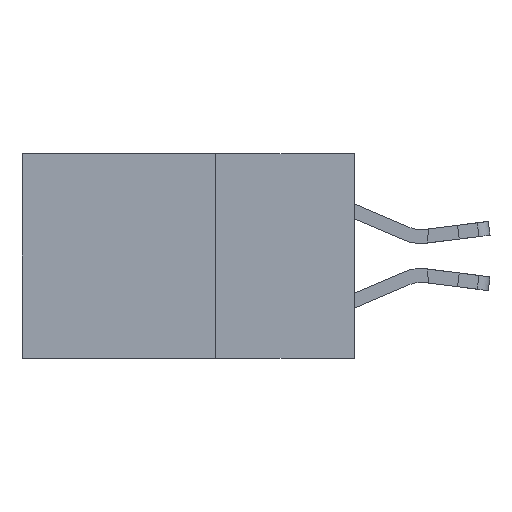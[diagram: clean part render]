
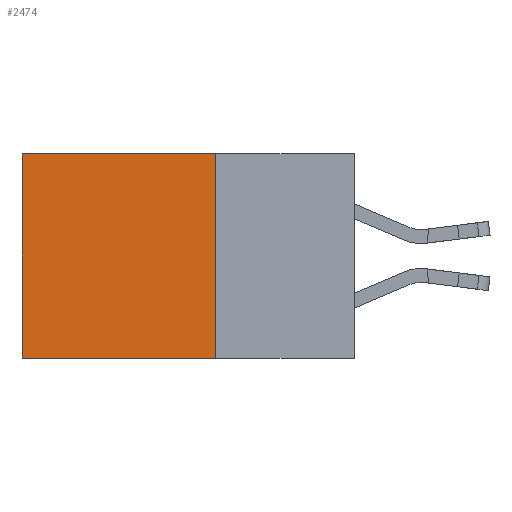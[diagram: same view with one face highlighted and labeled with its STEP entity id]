
A CAD part, left-side view. The second image highlights one B-rep face of the part: STEP entity #2474.
In plain terms, the highlighted planar face has unit normal (-1, 0, 0).
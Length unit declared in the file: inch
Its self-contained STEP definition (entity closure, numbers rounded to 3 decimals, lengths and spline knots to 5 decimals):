
#493 = CARTESIAN_POINT ( 'NONE',  ( 0.298, 0.25, 0. ) ) ;
#2474 = ADVANCED_FACE ( 'NONE', ( #22969 ), #17790, .F. ) ;
#2578 = VERTEX_POINT ( 'NONE', #23545 ) ;
#2821 = VERTEX_POINT ( 'NONE', #23646 ) ;
#2995 = DIRECTION ( 'NONE',  ( 0., 1., 0. ) ) ;
#3451 = AXIS2_PLACEMENT_3D ( 'NONE', #17655, #21585, #21608 ) ;
#4614 = ORIENTED_EDGE ( 'NONE', *, *, #14174, .F. ) ;
#4644 = DIRECTION ( 'NONE',  ( 0., 0., -1. ) ) ;
#5321 = CARTESIAN_POINT ( 'NONE',  ( 0.298, 0.25, 0. ) ) ;
#5442 = LINE ( 'NONE', #5321, #15656 ) ;
#6389 = VECTOR ( 'NONE', #17091, 39.37008 ) ;
#7253 = EDGE_CURVE ( 'NONE', #2821, #21787, #18313, .T. ) ;
#8786 = VECTOR ( 'NONE', #4644, 39.37008 ) ;
#9282 = EDGE_CURVE ( 'NONE', #15193, #2821, #17267, .T. ) ;
#11605 = EDGE_LOOP ( 'NONE', ( #11889, #17019, #4614, #24381 ) ) ;
#11856 = VECTOR ( 'NONE', #2995, 39.37008 ) ;
#11889 = ORIENTED_EDGE ( 'NONE', *, *, #7253, .T. ) ;
#12897 = CARTESIAN_POINT ( 'NONE',  ( 0.298, 0.25, 0. ) ) ;
#14174 = EDGE_CURVE ( 'NONE', #15193, #2578, #5442, .T. ) ;
#15193 = VERTEX_POINT ( 'NONE', #493 ) ;
#15656 = VECTOR ( 'NONE', #23726, 39.37008 ) ;
#16890 = CARTESIAN_POINT ( 'NONE',  ( 0.298, 0.6, 0. ) ) ;
#17019 = ORIENTED_EDGE ( 'NONE', *, *, #21479, .F. ) ;
#17091 = DIRECTION ( 'NONE',  ( 0., 1., 0. ) ) ;
#17267 = LINE ( 'NONE', #12897, #6389 ) ;
#17308 = LINE ( 'NONE', #25360, #11856 ) ;
#17655 = CARTESIAN_POINT ( 'NONE',  ( 0.298, 0.25, 0. ) ) ;
#17790 = PLANE ( 'NONE',  #3451 ) ;
#18162 = CARTESIAN_POINT ( 'NONE',  ( 0.298, 0.6, -0.37 ) ) ;
#18313 = LINE ( 'NONE', #16890, #8786 ) ;
#21479 = EDGE_CURVE ( 'NONE', #2578, #21787, #17308, .T. ) ;
#21585 = DIRECTION ( 'NONE',  ( 1., 0., 0. ) ) ;
#21608 = DIRECTION ( 'NONE',  ( 0., 0., -1. ) ) ;
#21787 = VERTEX_POINT ( 'NONE', #18162 ) ;
#22969 = FACE_OUTER_BOUND ( 'NONE', #11605, .T. ) ;
#23545 = CARTESIAN_POINT ( 'NONE',  ( 0.298, 0.25, -0.37 ) ) ;
#23646 = CARTESIAN_POINT ( 'NONE',  ( 0.298, 0.6, 0. ) ) ;
#23726 = DIRECTION ( 'NONE',  ( 0., 0., -1. ) ) ;
#24381 = ORIENTED_EDGE ( 'NONE', *, *, #9282, .T. ) ;
#25360 = CARTESIAN_POINT ( 'NONE',  ( 0.298, 0.25, -0.37 ) ) ;
